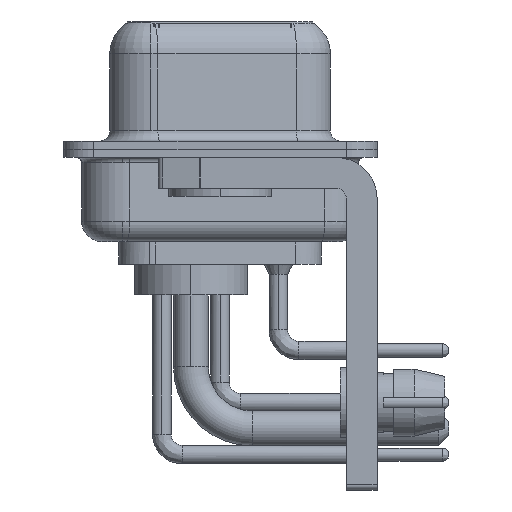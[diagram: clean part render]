
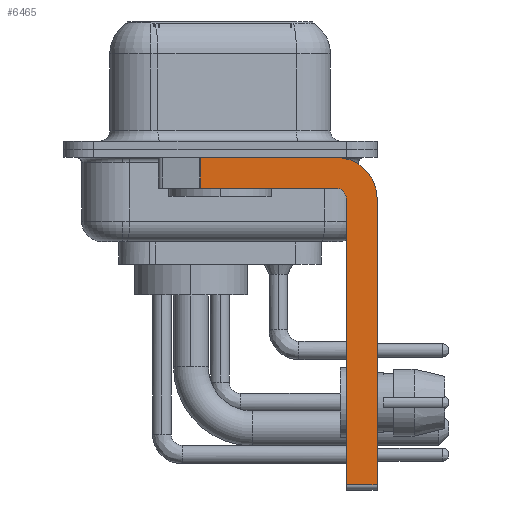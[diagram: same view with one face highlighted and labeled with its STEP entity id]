
A CAD part, left-side view. The second image highlights one B-rep face of the part: STEP entity #6465.
In plain terms, the highlighted planar face has unit normal (-1, 0, 0).
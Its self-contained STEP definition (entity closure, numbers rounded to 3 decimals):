
#320 = VERTEX_POINT ( 'NONE', #28476 ) ;
#776 = EDGE_CURVE ( 'NONE', #22060, #19468, #9390, .T. ) ;
#1890 = VECTOR ( 'NONE', #32338, 1000. ) ;
#1987 = EDGE_CURVE ( 'NONE', #22060, #10631, #31235, .T. ) ;
#3338 = DIRECTION ( 'NONE',  ( 0., 0., 1. ) ) ;
#3346 = LINE ( 'NONE', #11284, #23314 ) ;
#3379 = CIRCLE ( 'NONE', #23979, 0.5 ) ;
#4187 = EDGE_CURVE ( 'NONE', #19468, #30003, #3379, .T. ) ;
#5372 = VERTEX_POINT ( 'NONE', #16325 ) ;
#5470 = VERTEX_POINT ( 'NONE', #24620 ) ;
#6109 = DIRECTION ( 'NONE',  ( -1., 0., 0. ) ) ;
#6465 = ADVANCED_FACE ( 'NONE', ( #13871 ), #11107, .F. ) ;
#6475 = DIRECTION ( 'NONE',  ( 0., 1., 0. ) ) ;
#6962 = CARTESIAN_POINT ( 'NONE',  ( -2.9, -6.15, -2.4 ) ) ;
#8010 = CARTESIAN_POINT ( 'NONE',  ( -2.9, -7.65, -2.4 ) ) ;
#8443 = DIRECTION ( 'NONE',  ( 0., 0., -1. ) ) ;
#8890 = DIRECTION ( 'NONE',  ( 0., -1., 0. ) ) ;
#9390 = LINE ( 'NONE', #23049, #23024 ) ;
#10383 = CARTESIAN_POINT ( 'NONE',  ( -2.9, -6.15, -16.35 ) ) ;
#10390 = ORIENTED_EDGE ( 'NONE', *, *, #4187, .F. ) ;
#10631 = VERTEX_POINT ( 'NONE', #14037 ) ;
#10648 = DIRECTION ( 'NONE',  ( 1., 0., 0. ) ) ;
#11107 = PLANE ( 'NONE',  #28401 ) ;
#11125 = CARTESIAN_POINT ( 'NONE',  ( -2.9, 3., -0.4 ) ) ;
#11284 = CARTESIAN_POINT ( 'NONE',  ( -2.9, -5.65, -1.9 ) ) ;
#13521 = EDGE_CURVE ( 'NONE', #5470, #10631, #16863, .T. ) ;
#13871 = FACE_OUTER_BOUND ( 'NONE', #14154, .T. ) ;
#14037 = CARTESIAN_POINT ( 'NONE',  ( -2.9, -7.65, -16.35 ) ) ;
#14154 = EDGE_LOOP ( 'NONE', ( #25475, #30201, #32619, #10390, #18238, #18985, #14879, #35905 ) ) ;
#14756 = DIRECTION ( 'NONE',  ( 0., 0., 1. ) ) ;
#14879 = ORIENTED_EDGE ( 'NONE', *, *, #13521, .F. ) ;
#15512 = EDGE_CURVE ( 'NONE', #30003, #5372, #3346, .T. ) ;
#15526 = CIRCLE ( 'NONE', #36072, 2. ) ;
#16325 = CARTESIAN_POINT ( 'NONE',  ( -2.9, 0.978, -1.9 ) ) ;
#16863 = LINE ( 'NONE', #8010, #19877 ) ;
#17493 = CARTESIAN_POINT ( 'NONE',  ( -2.9, -5.65, -1.9 ) ) ;
#18238 = ORIENTED_EDGE ( 'NONE', *, *, #776, .F. ) ;
#18985 = ORIENTED_EDGE ( 'NONE', *, *, #1987, .T. ) ;
#19468 = VERTEX_POINT ( 'NONE', #6962 ) ;
#19487 = VECTOR ( 'NONE', #8443, 1000. ) ;
#19877 = VECTOR ( 'NONE', #30485, 1000. ) ;
#22060 = VERTEX_POINT ( 'NONE', #10383 ) ;
#22201 = CARTESIAN_POINT ( 'NONE',  ( -2.9, 0.978, -0.4 ) ) ;
#23024 = VECTOR ( 'NONE', #14756, 1000. ) ;
#23049 = CARTESIAN_POINT ( 'NONE',  ( -2.9, -6.15, -16.6 ) ) ;
#23079 = VECTOR ( 'NONE', #8890, 1000. ) ;
#23314 = VECTOR ( 'NONE', #6475, 1000. ) ;
#23609 = EDGE_CURVE ( 'NONE', #32068, #320, #36129, .T. ) ;
#23979 = AXIS2_PLACEMENT_3D ( 'NONE', #28594, #6109, #3338 ) ;
#24620 = CARTESIAN_POINT ( 'NONE',  ( -2.9, -7.65, -2.4 ) ) ;
#24655 = CARTESIAN_POINT ( 'NONE',  ( -2.9, -5.65, -2.4 ) ) ;
#25475 = ORIENTED_EDGE ( 'NONE', *, *, #23609, .F. ) ;
#27957 = DIRECTION ( 'NONE',  ( 0., 0., -1. ) ) ;
#27987 = LINE ( 'NONE', #36059, #19487 ) ;
#28401 = AXIS2_PLACEMENT_3D ( 'NONE', #33552, #30796, #34251 ) ;
#28476 = CARTESIAN_POINT ( 'NONE',  ( -2.9, -5.65, -0.4 ) ) ;
#28594 = CARTESIAN_POINT ( 'NONE',  ( -2.9, -5.65, -2.4 ) ) ;
#29945 = CARTESIAN_POINT ( 'NONE',  ( -2.9, -5.65, -16.35 ) ) ;
#30003 = VERTEX_POINT ( 'NONE', #17493 ) ;
#30201 = ORIENTED_EDGE ( 'NONE', *, *, #35289, .T. ) ;
#30243 = EDGE_CURVE ( 'NONE', #320, #5470, #15526, .T. ) ;
#30485 = DIRECTION ( 'NONE',  ( 0., 0., -1. ) ) ;
#30796 = DIRECTION ( 'NONE',  ( 1., 0., 0. ) ) ;
#31235 = LINE ( 'NONE', #29945, #1890 ) ;
#32068 = VERTEX_POINT ( 'NONE', #22201 ) ;
#32338 = DIRECTION ( 'NONE',  ( 0., -1., 0. ) ) ;
#32619 = ORIENTED_EDGE ( 'NONE', *, *, #15512, .F. ) ;
#33552 = CARTESIAN_POINT ( 'NONE',  ( -2.9, -5.65, -2.4 ) ) ;
#34251 = DIRECTION ( 'NONE',  ( 0., 0., -1. ) ) ;
#35289 = EDGE_CURVE ( 'NONE', #32068, #5372, #27987, .T. ) ;
#35905 = ORIENTED_EDGE ( 'NONE', *, *, #30243, .F. ) ;
#36059 = CARTESIAN_POINT ( 'NONE',  ( -2.9, 0.978, -1.9 ) ) ;
#36072 = AXIS2_PLACEMENT_3D ( 'NONE', #24655, #10648, #27957 ) ;
#36129 = LINE ( 'NONE', #11125, #23079 ) ;
